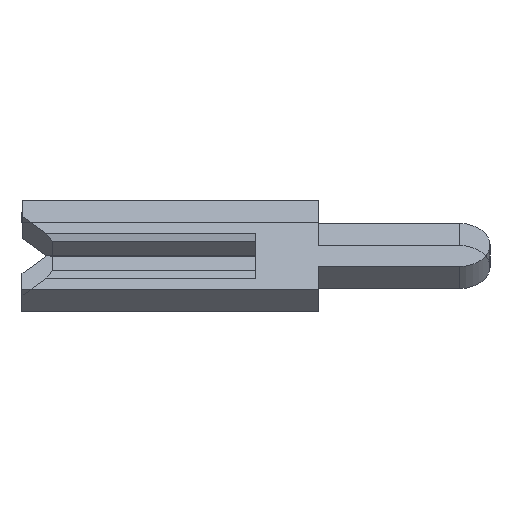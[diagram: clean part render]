
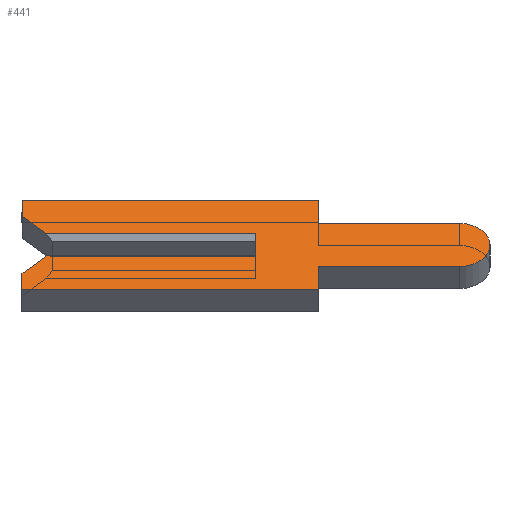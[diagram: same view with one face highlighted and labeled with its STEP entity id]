
A CAD part, left-side view. The second image highlights one B-rep face of the part: STEP entity #441.
In plain terms, the highlighted face is planar.
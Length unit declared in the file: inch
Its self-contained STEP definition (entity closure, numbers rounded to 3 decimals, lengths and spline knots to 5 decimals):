
#10 = LINE ( 'NONE', #1491, #2377 ) ;
#24 = AXIS2_PLACEMENT_3D ( 'NONE', #2361, #1926, #1064 ) ;
#26 = DIRECTION ( 'NONE',  ( 0., 0., 1. ) ) ;
#52 = EDGE_CURVE ( 'NONE', #458, #1245, #10, .T. ) ;
#64 = CARTESIAN_POINT ( 'NONE',  ( -0.01, -0.1305, 0. ) ) ;
#74 = VECTOR ( 'NONE', #1548, 39.37008 ) ;
#102 = CARTESIAN_POINT ( 'NONE',  ( -0.01, -0.1305, 0.0195 ) ) ;
#113 = CARTESIAN_POINT ( 'NONE',  ( -0.01, 0.15, 0.04 ) ) ;
#134 = LINE ( 'NONE', #545, #2284 ) ;
#185 = VECTOR ( 'NONE', #2050, 39.37008 ) ;
#213 = VECTOR ( 'NONE', #1817, 39.37008 ) ;
#219 = VERTEX_POINT ( 'NONE', #838 ) ;
#249 = ORIENTED_EDGE ( 'NONE', *, *, #1542, .F. ) ;
#268 = CARTESIAN_POINT ( 'NONE',  ( -0.01, 0.15, -0.026 ) ) ;
#275 = CIRCLE ( 'NONE', #24, 0.0195 ) ;
#278 = DIRECTION ( 'NONE',  ( 1., 0., 0. ) ) ;
#289 = VERTEX_POINT ( 'NONE', #1943 ) ;
#313 = CARTESIAN_POINT ( 'NONE',  ( -0.01, -0.04, 0.0195 ) ) ;
#335 = CARTESIAN_POINT ( 'NONE',  ( -0.01, 0.134, -0.01 ) ) ;
#350 = CARTESIAN_POINT ( 'NONE',  ( -0.01, -0.04, -0.0195 ) ) ;
#359 = CARTESIAN_POINT ( 'NONE',  ( -0.01, -0.04, -0.04 ) ) ;
#383 = ORIENTED_EDGE ( 'NONE', *, *, #1389, .F. ) ;
#398 = VERTEX_POINT ( 'NONE', #268 ) ;
#441 = ADVANCED_FACE ( 'NONE', ( #2226 ), #1738, .F. ) ;
#443 = LINE ( 'NONE', #593, #2055 ) ;
#458 = VERTEX_POINT ( 'NONE', #702 ) ;
#489 = ORIENTED_EDGE ( 'NONE', *, *, #1948, .F. ) ;
#545 = CARTESIAN_POINT ( 'NONE',  ( -0.01, -0.04, 0.0195 ) ) ;
#574 = VERTEX_POINT ( 'NONE', #102 ) ;
#593 = CARTESIAN_POINT ( 'NONE',  ( -0.01, 0., 0.0065 ) ) ;
#628 = DIRECTION ( 'NONE',  ( 0., 1., 0. ) ) ;
#642 = EDGE_CURVE ( 'NONE', #1039, #398, #909, .T. ) ;
#667 = ORIENTED_EDGE ( 'NONE', *, *, #2645, .F. ) ;
#702 = CARTESIAN_POINT ( 'NONE',  ( -0.01, -0.04, 0.04 ) ) ;
#707 = CARTESIAN_POINT ( 'NONE',  ( -0.01, -0.1305, -0.01 ) ) ;
#723 = CARTESIAN_POINT ( 'NONE',  ( -0.01, 0.15, -0.04 ) ) ;
#745 = LINE ( 'NONE', #1790, #185 ) ;
#750 = DIRECTION ( 'NONE',  ( 0., -1., 0. ) ) ;
#755 = CARTESIAN_POINT ( 'NONE',  ( -0.01, 0.15, 0.026 ) ) ;
#776 = LINE ( 'NONE', #2041, #2095 ) ;
#779 = ORIENTED_EDGE ( 'NONE', *, *, #52, .F. ) ;
#835 = DIRECTION ( 'NONE',  ( 0., -1., 0. ) ) ;
#838 = CARTESIAN_POINT ( 'NONE',  ( -0.01, 0., 0.01 ) ) ;
#839 = ORIENTED_EDGE ( 'NONE', *, *, #1693, .F. ) ;
#909 = LINE ( 'NONE', #2559, #74 ) ;
#910 = VERTEX_POINT ( 'NONE', #113 ) ;
#936 = LINE ( 'NONE', #707, #1780 ) ;
#991 = EDGE_CURVE ( 'NONE', #910, #458, #1617, .T. ) ;
#1039 = VERTEX_POINT ( 'NONE', #723 ) ;
#1043 = CARTESIAN_POINT ( 'NONE',  ( -0.01, 0.15, 0.026 ) ) ;
#1064 = DIRECTION ( 'NONE',  ( 0., 0., -1. ) ) ;
#1170 = VECTOR ( 'NONE', #835, 39.37008 ) ;
#1222 = CARTESIAN_POINT ( 'NONE',  ( -0.01, 0.15, 0.01 ) ) ;
#1229 = CARTESIAN_POINT ( 'NONE',  ( -0.01, 0., -0.01 ) ) ;
#1245 = VERTEX_POINT ( 'NONE', #313 ) ;
#1262 = EDGE_LOOP ( 'NONE', ( #2634, #489, #667, #2067, #2614, #1414, #383, #839, #2169, #2273, #779, #1386, #1918, #249 ) ) ;
#1304 = VECTOR ( 'NONE', #26, 39.37008 ) ;
#1324 = AXIS2_PLACEMENT_3D ( 'NONE', #64, #278, #1953 ) ;
#1386 = ORIENTED_EDGE ( 'NONE', *, *, #991, .F. ) ;
#1389 = EDGE_CURVE ( 'NONE', #1824, #1497, #776, .T. ) ;
#1414 = ORIENTED_EDGE ( 'NONE', *, *, #2454, .F. ) ;
#1491 = CARTESIAN_POINT ( 'NONE',  ( -0.01, -0.04, 0.04 ) ) ;
#1497 = VERTEX_POINT ( 'NONE', #359 ) ;
#1534 = CARTESIAN_POINT ( 'NONE',  ( -0.01, -0.1305, -0.0195 ) ) ;
#1542 = EDGE_CURVE ( 'NONE', #289, #1913, #2420, .T. ) ;
#1548 = DIRECTION ( 'NONE',  ( 0., 0., 1. ) ) ;
#1560 = LINE ( 'NONE', #350, #213 ) ;
#1584 = VECTOR ( 'NONE', #628, 39.37008 ) ;
#1605 = EDGE_CURVE ( 'NONE', #398, #1729, #745, .T. ) ;
#1617 = LINE ( 'NONE', #2632, #1648 ) ;
#1648 = VECTOR ( 'NONE', #750, 39.37008 ) ;
#1693 = EDGE_CURVE ( 'NONE', #2629, #1824, #1560, .T. ) ;
#1722 = LINE ( 'NONE', #1222, #1170 ) ;
#1729 = VERTEX_POINT ( 'NONE', #335 ) ;
#1738 = PLANE ( 'NONE',  #1324 ) ;
#1780 = VECTOR ( 'NONE', #1977, 39.37008 ) ;
#1790 = CARTESIAN_POINT ( 'NONE',  ( -0.01, 0.1305, -0.0065 ) ) ;
#1813 = EDGE_CURVE ( 'NONE', #1245, #574, #134, .T. ) ;
#1817 = DIRECTION ( 'NONE',  ( 0., 1., 0. ) ) ;
#1824 = VERTEX_POINT ( 'NONE', #2093 ) ;
#1840 = LINE ( 'NONE', #755, #1304 ) ;
#1882 = CARTESIAN_POINT ( 'NONE',  ( -0.01, 0.15, -0.04 ) ) ;
#1888 = VERTEX_POINT ( 'NONE', #1229 ) ;
#1913 = VERTEX_POINT ( 'NONE', #1043 ) ;
#1918 = ORIENTED_EDGE ( 'NONE', *, *, #2096, .F. ) ;
#1926 = DIRECTION ( 'NONE',  ( 1., 0., 0. ) ) ;
#1943 = CARTESIAN_POINT ( 'NONE',  ( -0.01, 0.134, 0.01 ) ) ;
#1948 = EDGE_CURVE ( 'NONE', #1888, #219, #443, .T. ) ;
#1953 = DIRECTION ( 'NONE',  ( 0., 0., -1. ) ) ;
#1977 = DIRECTION ( 'NONE',  ( 0., -1., 0. ) ) ;
#2041 = CARTESIAN_POINT ( 'NONE',  ( -0.01, -0.04, -0.04 ) ) ;
#2050 = DIRECTION ( 'NONE',  ( 0., -0.707, 0.707 ) ) ;
#2055 = VECTOR ( 'NONE', #2486, 39.37008 ) ;
#2067 = ORIENTED_EDGE ( 'NONE', *, *, #1605, .F. ) ;
#2070 = EDGE_CURVE ( 'NONE', #289, #219, #1722, .T. ) ;
#2093 = CARTESIAN_POINT ( 'NONE',  ( -0.01, -0.04, -0.0195 ) ) ;
#2095 = VECTOR ( 'NONE', #2238, 39.37008 ) ;
#2096 = EDGE_CURVE ( 'NONE', #1913, #910, #1840, .T. ) ;
#2100 = DIRECTION ( 'NONE',  ( 0., -1., 0. ) ) ;
#2169 = ORIENTED_EDGE ( 'NONE', *, *, #2214, .F. ) ;
#2186 = DIRECTION ( 'NONE',  ( 0., 0.707, 0.707 ) ) ;
#2214 = EDGE_CURVE ( 'NONE', #574, #2629, #275, .T. ) ;
#2226 = FACE_OUTER_BOUND ( 'NONE', #1262, .T. ) ;
#2238 = DIRECTION ( 'NONE',  ( 0., 0., -1. ) ) ;
#2273 = ORIENTED_EDGE ( 'NONE', *, *, #1813, .F. ) ;
#2284 = VECTOR ( 'NONE', #2100, 39.37008 ) ;
#2335 = DIRECTION ( 'NONE',  ( 0., 0., -1. ) ) ;
#2356 = LINE ( 'NONE', #1882, #1584 ) ;
#2361 = CARTESIAN_POINT ( 'NONE',  ( -0.01, -0.1305, 0. ) ) ;
#2377 = VECTOR ( 'NONE', #2335, 39.37008 ) ;
#2420 = LINE ( 'NONE', #2510, #2561 ) ;
#2454 = EDGE_CURVE ( 'NONE', #1497, #1039, #2356, .T. ) ;
#2486 = DIRECTION ( 'NONE',  ( 0., 0., 1. ) ) ;
#2510 = CARTESIAN_POINT ( 'NONE',  ( -0.01, 0.1305, 0.0065 ) ) ;
#2559 = CARTESIAN_POINT ( 'NONE',  ( -0.01, 0.15, -0.026 ) ) ;
#2561 = VECTOR ( 'NONE', #2186, 39.37008 ) ;
#2614 = ORIENTED_EDGE ( 'NONE', *, *, #642, .F. ) ;
#2629 = VERTEX_POINT ( 'NONE', #1534 ) ;
#2632 = CARTESIAN_POINT ( 'NONE',  ( -0.01, 0.15, 0.04 ) ) ;
#2634 = ORIENTED_EDGE ( 'NONE', *, *, #2070, .T. ) ;
#2645 = EDGE_CURVE ( 'NONE', #1729, #1888, #936, .T. ) ;
